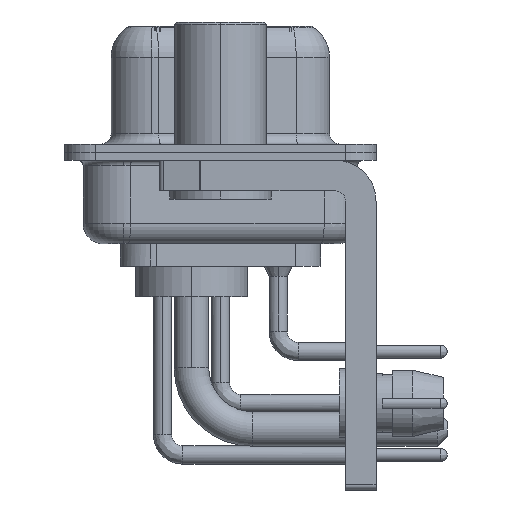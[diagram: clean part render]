
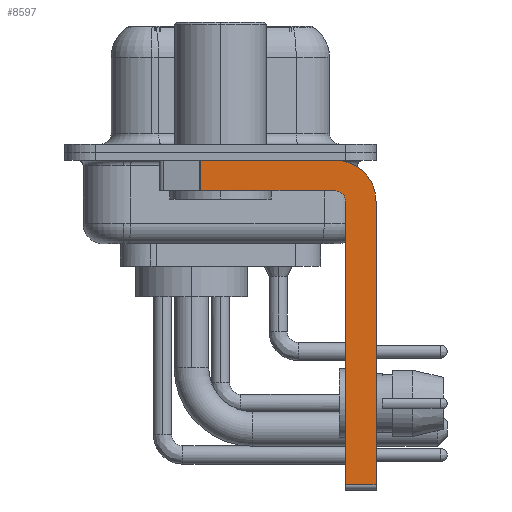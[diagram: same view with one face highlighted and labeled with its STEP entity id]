
A CAD part, left-side view. The second image highlights one B-rep face of the part: STEP entity #8597.
In plain terms, the highlighted planar face has unit normal (-1, 0, 0).
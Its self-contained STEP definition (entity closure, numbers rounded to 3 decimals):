
#562 = CARTESIAN_POINT ( 'NONE',  ( -2.9, 0.978, -1.9 ) ) ;
#936 = VECTOR ( 'NONE', #16013, 1000. ) ;
#1011 = LINE ( 'NONE', #28818, #936 ) ;
#1419 = DIRECTION ( 'NONE',  ( 1., 0., 0. ) ) ;
#1515 = VERTEX_POINT ( 'NONE', #16529 ) ;
#1758 = ORIENTED_EDGE ( 'NONE', *, *, #9240, .F. ) ;
#1883 = EDGE_CURVE ( 'NONE', #13577, #4228, #29620, .T. ) ;
#2118 = EDGE_CURVE ( 'NONE', #15891, #1515, #14496, .T. ) ;
#2640 = VERTEX_POINT ( 'NONE', #12594 ) ;
#2750 = LINE ( 'NONE', #20265, #11463 ) ;
#3073 = CIRCLE ( 'NONE', #7327, 2. ) ;
#3531 = VERTEX_POINT ( 'NONE', #10289 ) ;
#4228 = VERTEX_POINT ( 'NONE', #15744 ) ;
#4393 = LINE ( 'NONE', #14546, #11422 ) ;
#7049 = DIRECTION ( 'NONE',  ( 0., -1., 0. ) ) ;
#7327 = AXIS2_PLACEMENT_3D ( 'NONE', #16737, #11739, #11406 ) ;
#8597 = ADVANCED_FACE ( 'NONE', ( #32020 ), #31526, .F. ) ;
#8630 = AXIS2_PLACEMENT_3D ( 'NONE', #22475, #30415, #17302 ) ;
#9240 = EDGE_CURVE ( 'NONE', #23552, #3531, #4393, .T. ) ;
#10289 = CARTESIAN_POINT ( 'NONE',  ( -2.9, -5.65, -0.4 ) ) ;
#11406 = DIRECTION ( 'NONE',  ( 0., 0., -1. ) ) ;
#11422 = VECTOR ( 'NONE', #7049, 1000. ) ;
#11463 = VECTOR ( 'NONE', #19937, 1000. ) ;
#11739 = DIRECTION ( 'NONE',  ( 1., 0., 0. ) ) ;
#11765 = CARTESIAN_POINT ( 'NONE',  ( -2.9, -5.65, -2.4 ) ) ;
#11830 = DIRECTION ( 'NONE',  ( 0., 0., -1. ) ) ;
#12594 = CARTESIAN_POINT ( 'NONE',  ( -2.9, -6.15, -16.35 ) ) ;
#13245 = CARTESIAN_POINT ( 'NONE',  ( -2.9, -5.65, -16.35 ) ) ;
#13577 = VERTEX_POINT ( 'NONE', #25677 ) ;
#14100 = DIRECTION ( 'NONE',  ( 0., 0., -1. ) ) ;
#14475 = EDGE_CURVE ( 'NONE', #2640, #15891, #2750, .T. ) ;
#14496 = CIRCLE ( 'NONE', #8630, 0.5 ) ;
#14546 = CARTESIAN_POINT ( 'NONE',  ( -2.9, 3., -0.4 ) ) ;
#14691 = ORIENTED_EDGE ( 'NONE', *, *, #32566, .T. ) ;
#15744 = CARTESIAN_POINT ( 'NONE',  ( -2.9, -7.65, -16.35 ) ) ;
#15891 = VERTEX_POINT ( 'NONE', #30650 ) ;
#16013 = DIRECTION ( 'NONE',  ( 0., 1., 0. ) ) ;
#16529 = CARTESIAN_POINT ( 'NONE',  ( -2.9, -5.65, -1.9 ) ) ;
#16706 = ORIENTED_EDGE ( 'NONE', *, *, #17674, .F. ) ;
#16737 = CARTESIAN_POINT ( 'NONE',  ( -2.9, -5.65, -2.4 ) ) ;
#17302 = DIRECTION ( 'NONE',  ( 0., 0., 1. ) ) ;
#17361 = ORIENTED_EDGE ( 'NONE', *, *, #2118, .F. ) ;
#17674 = EDGE_CURVE ( 'NONE', #1515, #27368, #1011, .T. ) ;
#19022 = ORIENTED_EDGE ( 'NONE', *, *, #1883, .F. ) ;
#19937 = DIRECTION ( 'NONE',  ( 0., 0., 1. ) ) ;
#20265 = CARTESIAN_POINT ( 'NONE',  ( -2.9, -6.15, -16.6 ) ) ;
#20278 = VECTOR ( 'NONE', #27647, 1000. ) ;
#22475 = CARTESIAN_POINT ( 'NONE',  ( -2.9, -5.65, -2.4 ) ) ;
#23333 = CARTESIAN_POINT ( 'NONE',  ( -2.9, 0.978, -0.4 ) ) ;
#23480 = EDGE_CURVE ( 'NONE', #23552, #27368, #30283, .T. ) ;
#23552 = VERTEX_POINT ( 'NONE', #23333 ) ;
#23821 = ORIENTED_EDGE ( 'NONE', *, *, #23480, .T. ) ;
#24080 = AXIS2_PLACEMENT_3D ( 'NONE', #11765, #1419, #14100 ) ;
#24497 = CARTESIAN_POINT ( 'NONE',  ( -2.9, -7.65, -2.4 ) ) ;
#25677 = CARTESIAN_POINT ( 'NONE',  ( -2.9, -7.65, -2.4 ) ) ;
#25902 = LINE ( 'NONE', #13245, #29668 ) ;
#27368 = VERTEX_POINT ( 'NONE', #562 ) ;
#27647 = DIRECTION ( 'NONE',  ( 0., 0., -1. ) ) ;
#27751 = ORIENTED_EDGE ( 'NONE', *, *, #14475, .F. ) ;
#28176 = EDGE_LOOP ( 'NONE', ( #1758, #23821, #16706, #17361, #27751, #14691, #19022, #29753 ) ) ;
#28391 = DIRECTION ( 'NONE',  ( 0., -1., 0. ) ) ;
#28818 = CARTESIAN_POINT ( 'NONE',  ( -2.9, -5.65, -1.9 ) ) ;
#29620 = LINE ( 'NONE', #24497, #29875 ) ;
#29668 = VECTOR ( 'NONE', #28391, 1000. ) ;
#29753 = ORIENTED_EDGE ( 'NONE', *, *, #32796, .F. ) ;
#29875 = VECTOR ( 'NONE', #11830, 1000. ) ;
#30115 = CARTESIAN_POINT ( 'NONE',  ( -2.9, 0.978, -1.9 ) ) ;
#30283 = LINE ( 'NONE', #30115, #20278 ) ;
#30415 = DIRECTION ( 'NONE',  ( -1., 0., 0. ) ) ;
#30650 = CARTESIAN_POINT ( 'NONE',  ( -2.9, -6.15, -2.4 ) ) ;
#31526 = PLANE ( 'NONE',  #24080 ) ;
#32020 = FACE_OUTER_BOUND ( 'NONE', #28176, .T. ) ;
#32566 = EDGE_CURVE ( 'NONE', #2640, #4228, #25902, .T. ) ;
#32796 = EDGE_CURVE ( 'NONE', #3531, #13577, #3073, .T. ) ;
